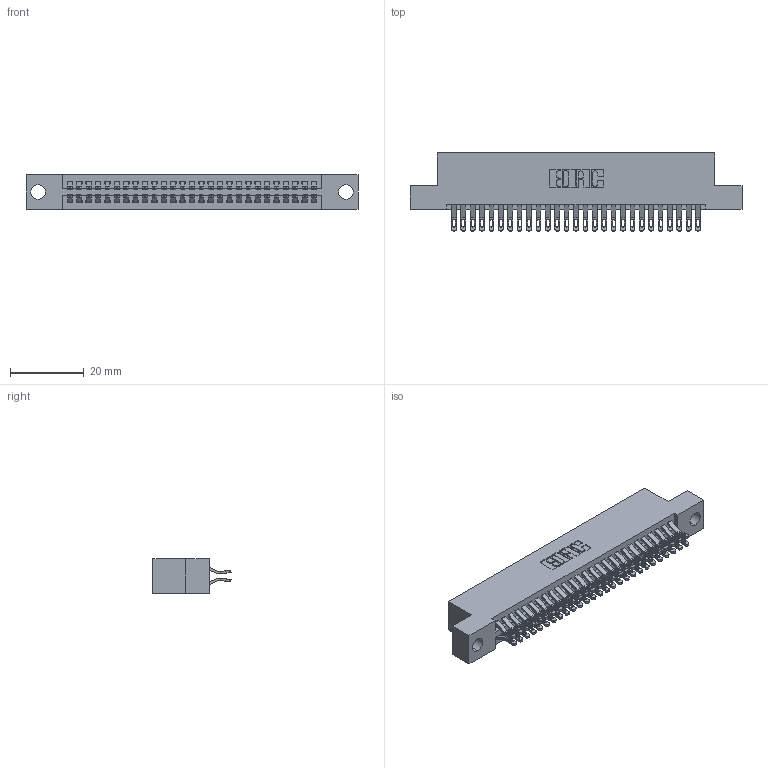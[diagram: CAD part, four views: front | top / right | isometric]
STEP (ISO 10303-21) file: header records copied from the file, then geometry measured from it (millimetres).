
FILE_DESCRIPTION (( 'STEP AP203' ), '1' );
FILE_NAME ('345-054-555-204.STEP', '2021-05-20T04:14:47', ( '' ), ( '' ), 'SwSTEP 2.0', 'SolidWorks 2020', '' );
FILE_SCHEMA (( 'CONFIG_CONTROL_DESIGN' ));
Length unit declared in the file: inch
Products named in the file (3): 345-292-001_555 Tail; 345-054-555-204; 345 Part_Flush Mounting Lugs - 0.156 Dia-TI
Assembly tree (55 placements, depth 2):
  345-054-555-204
    345 Part_Flush Mounting Lugs - 0.156 Dia-TI
    345-292-001_555 Tail  x54
Bounding box: 89.79 x 21.13 x 9.4 mm (x, y, z)
Volume: 8633.6 mm3; surface area: 12867.8 mm2
Topology: 55 solids, 55 shells, 3164 faces, 9935 edges, 6622 vertices
Faces by surface type: plane 1768, cylinder 1396
Entity records: 23949 total; most frequent: CARTESIAN_POINT 4068, ORIENTED_EDGE 3970, DIRECTION 3573, EDGE_CURVE 1985, VECTOR 1725, LINE 1725, VERTEX_POINT 1322, AXIS2_PLACEMENT_3D 924
